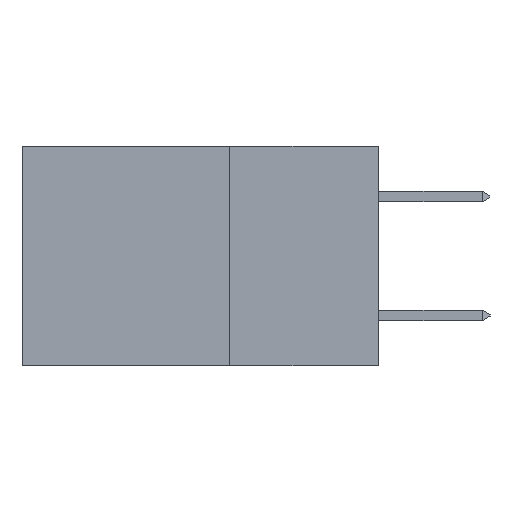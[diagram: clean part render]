
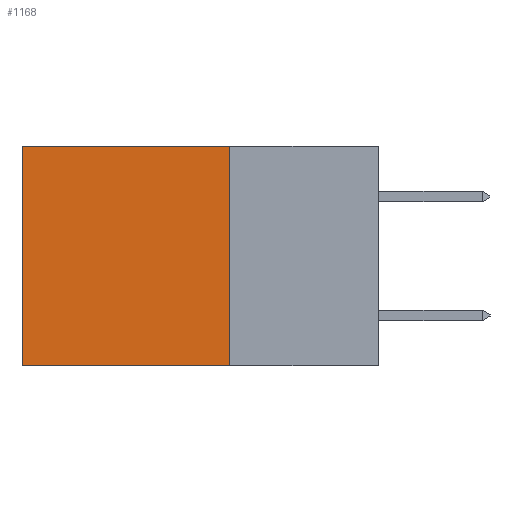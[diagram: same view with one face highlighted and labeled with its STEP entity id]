
A CAD part, left-side view. The second image highlights one B-rep face of the part: STEP entity #1168.
In plain terms, the highlighted planar face has unit normal (-1, 0, 0).
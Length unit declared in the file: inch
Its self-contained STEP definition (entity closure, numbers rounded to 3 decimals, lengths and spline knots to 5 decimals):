
#259 = VERTEX_POINT ( 'NONE', #14383 ) ;
#1090 = ORIENTED_EDGE ( 'NONE', *, *, #16063, .T. ) ;
#1168 = ADVANCED_FACE ( 'NONE', ( #25281 ), #18809, .F. ) ;
#1280 = CARTESIAN_POINT ( 'NONE',  ( 0.2615, 0.25, -0.37 ) ) ;
#2221 = DIRECTION ( 'NONE',  ( 0., 1., 0. ) ) ;
#2603 = LINE ( 'NONE', #1280, #12178 ) ;
#2784 = VECTOR ( 'NONE', #25611, 39.37008 ) ;
#4183 = CARTESIAN_POINT ( 'NONE',  ( 0.2615, 0.6, 0. ) ) ;
#4860 = VECTOR ( 'NONE', #2221, 39.37008 ) ;
#7054 = CARTESIAN_POINT ( 'NONE',  ( 0.2615, 0.25, -0.37 ) ) ;
#7978 = VERTEX_POINT ( 'NONE', #7054 ) ;
#8616 = CARTESIAN_POINT ( 'NONE',  ( 0.2615, 0.25, 0. ) ) ;
#9090 = VERTEX_POINT ( 'NONE', #4183 ) ;
#9417 = DIRECTION ( 'NONE',  ( 0., 1., 0. ) ) ;
#9536 = EDGE_CURVE ( 'NONE', #9090, #259, #24220, .T. ) ;
#9995 = CARTESIAN_POINT ( 'NONE',  ( 0.2615, 0.6, -0.37 ) ) ;
#12178 = VECTOR ( 'NONE', #9417, 39.37008 ) ;
#13186 = EDGE_CURVE ( 'NONE', #15732, #7978, #24750, .T. ) ;
#14383 = CARTESIAN_POINT ( 'NONE',  ( 0.2615, 0.6, -0.37 ) ) ;
#15049 = ORIENTED_EDGE ( 'NONE', *, *, #16442, .F. ) ;
#15132 = CARTESIAN_POINT ( 'NONE',  ( 0.2615, 0.25, -0.37 ) ) ;
#15732 = VERTEX_POINT ( 'NONE', #8616 ) ;
#16063 = EDGE_CURVE ( 'NONE', #15732, #9090, #21355, .T. ) ;
#16442 = EDGE_CURVE ( 'NONE', #7978, #259, #2603, .T. ) ;
#18291 = DIRECTION ( 'NONE',  ( 0., 0., -1. ) ) ;
#18804 = CARTESIAN_POINT ( 'NONE',  ( 0.2615, 0.25, -0.37 ) ) ;
#18809 = PLANE ( 'NONE',  #26532 ) ;
#19358 = DIRECTION ( 'NONE',  ( 1., 0., 0. ) ) ;
#21355 = LINE ( 'NONE', #24895, #4860 ) ;
#22926 = VECTOR ( 'NONE', #24540, 39.37008 ) ;
#24220 = LINE ( 'NONE', #9995, #22926 ) ;
#24222 = ORIENTED_EDGE ( 'NONE', *, *, #9536, .T. ) ;
#24540 = DIRECTION ( 'NONE',  ( 0., 0., -1. ) ) ;
#24750 = LINE ( 'NONE', #15132, #2784 ) ;
#24895 = CARTESIAN_POINT ( 'NONE',  ( 0.2615, 0.25, 0. ) ) ;
#25281 = FACE_OUTER_BOUND ( 'NONE', #26008, .T. ) ;
#25611 = DIRECTION ( 'NONE',  ( 0., 0., -1. ) ) ;
#25891 = ORIENTED_EDGE ( 'NONE', *, *, #13186, .F. ) ;
#26008 = EDGE_LOOP ( 'NONE', ( #24222, #15049, #25891, #1090 ) ) ;
#26532 = AXIS2_PLACEMENT_3D ( 'NONE', #18804, #19358, #18291 ) ;
